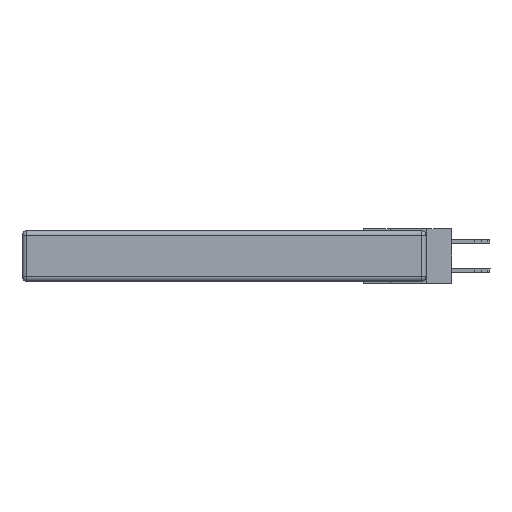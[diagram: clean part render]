
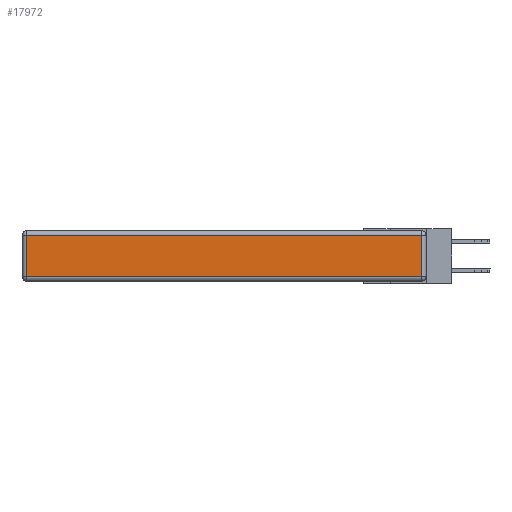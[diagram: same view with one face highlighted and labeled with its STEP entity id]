
A CAD part, left-side view. The second image highlights one B-rep face of the part: STEP entity #17972.
In plain terms, the highlighted planar face has unit normal (-1, 0, 0).
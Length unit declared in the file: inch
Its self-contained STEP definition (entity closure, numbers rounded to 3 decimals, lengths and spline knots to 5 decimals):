
#270 = VECTOR ( 'NONE', #23812, 39.37008 ) ;
#1841 = DIRECTION ( 'NONE',  ( 0., 0., 1. ) ) ;
#3194 = DIRECTION ( 'NONE',  ( 0., -1., 0. ) ) ;
#5631 = LINE ( 'NONE', #17670, #270 ) ;
#6159 = DIRECTION ( 'NONE',  ( 0., 0., -1. ) ) ;
#6524 = CARTESIAN_POINT ( 'NONE',  ( 0., 0.03, -0.03 ) ) ;
#7183 = VECTOR ( 'NONE', #6159, 39.37008 ) ;
#7861 = DIRECTION ( 'NONE',  ( -1., 0., 0. ) ) ;
#9400 = VERTEX_POINT ( 'NONE', #12753 ) ;
#11072 = VERTEX_POINT ( 'NONE', #20307 ) ;
#11244 = EDGE_CURVE ( 'NONE', #12987, #26281, #25605, .T. ) ;
#11897 = ORIENTED_EDGE ( 'NONE', *, *, #19828, .T. ) ;
#12753 = CARTESIAN_POINT ( 'NONE',  ( 0., 2.72, -0.313 ) ) ;
#12849 = ORIENTED_EDGE ( 'NONE', *, *, #19099, .T. ) ;
#12987 = VERTEX_POINT ( 'NONE', #6524 ) ;
#14145 = ORIENTED_EDGE ( 'NONE', *, *, #11244, .T. ) ;
#16007 = CARTESIAN_POINT ( 'NONE',  ( 0., 2.75, -0.03 ) ) ;
#16268 = FACE_OUTER_BOUND ( 'NONE', #23843, .T. ) ;
#17336 = VECTOR ( 'NONE', #26063, 39.37008 ) ;
#17670 = CARTESIAN_POINT ( 'NONE',  ( 0., 0.03, -0.343 ) ) ;
#17972 = ADVANCED_FACE ( 'NONE', ( #16268 ), #20267, .T. ) ;
#18707 = LINE ( 'NONE', #20275, #7183 ) ;
#18783 = LINE ( 'NONE', #23574, #21926 ) ;
#19099 = EDGE_CURVE ( 'NONE', #9400, #11072, #18783, .T. ) ;
#19828 = EDGE_CURVE ( 'NONE', #11072, #12987, #5631, .T. ) ;
#20267 = PLANE ( 'NONE',  #24393 ) ;
#20275 = CARTESIAN_POINT ( 'NONE',  ( 0., 2.72, -0.343 ) ) ;
#20307 = CARTESIAN_POINT ( 'NONE',  ( 0., 0.03, -0.313 ) ) ;
#20350 = ORIENTED_EDGE ( 'NONE', *, *, #22707, .T. ) ;
#21926 = VECTOR ( 'NONE', #3194, 39.37008 ) ;
#22707 = EDGE_CURVE ( 'NONE', #26281, #9400, #18707, .T. ) ;
#23574 = CARTESIAN_POINT ( 'NONE',  ( 0., 0., -0.313 ) ) ;
#23708 = CARTESIAN_POINT ( 'NONE',  ( 0., 2.72, -0.03 ) ) ;
#23812 = DIRECTION ( 'NONE',  ( 0., 0., 1. ) ) ;
#23843 = EDGE_LOOP ( 'NONE', ( #12849, #11897, #14145, #20350 ) ) ;
#24266 = CARTESIAN_POINT ( 'NONE',  ( 0., 0., -0.343 ) ) ;
#24393 = AXIS2_PLACEMENT_3D ( 'NONE', #24266, #7861, #1841 ) ;
#25605 = LINE ( 'NONE', #16007, #17336 ) ;
#26063 = DIRECTION ( 'NONE',  ( 0., 1., 0. ) ) ;
#26281 = VERTEX_POINT ( 'NONE', #23708 ) ;
